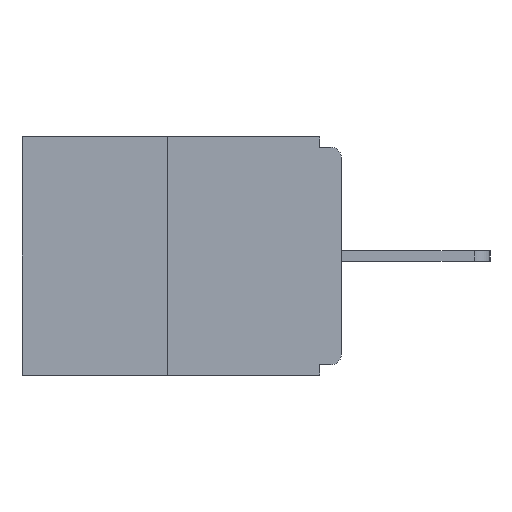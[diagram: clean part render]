
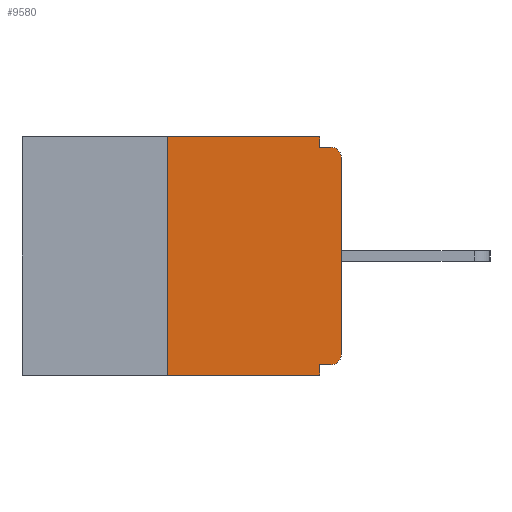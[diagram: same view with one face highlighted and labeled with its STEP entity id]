
A CAD part, left-side view. The second image highlights one B-rep face of the part: STEP entity #9580.
In plain terms, the highlighted planar face has unit normal (-1, 0, 0).
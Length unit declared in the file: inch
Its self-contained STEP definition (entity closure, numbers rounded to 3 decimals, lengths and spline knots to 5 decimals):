
#209 = DIRECTION ( 'NONE',  ( 0., 0., -1. ) ) ;
#618 = CIRCLE ( 'NONE', #10416, 0.015 ) ;
#1016 = CARTESIAN_POINT ( 'NONE',  ( 0., 0.25, 0. ) ) ;
#1125 = VERTEX_POINT ( 'NONE', #4318 ) ;
#2006 = VERTEX_POINT ( 'NONE', #5354 ) ;
#2096 = VECTOR ( 'NONE', #12347, 39.37008 ) ;
#3022 = CARTESIAN_POINT ( 'NONE',  ( 0., 0.015, -0.03 ) ) ;
#3151 = EDGE_CURVE ( 'NONE', #7987, #12108, #8639, .T. ) ;
#3240 = VECTOR ( 'NONE', #10092, 39.37008 ) ;
#3279 = CARTESIAN_POINT ( 'NONE',  ( 0., 0.46, 0. ) ) ;
#3523 = VECTOR ( 'NONE', #9205, 39.37008 ) ;
#3609 = VERTEX_POINT ( 'NONE', #15906 ) ;
#3686 = CIRCLE ( 'NONE', #14062, 0.015 ) ;
#3848 = DIRECTION ( 'NONE',  ( 0., 0., 1. ) ) ;
#3893 = EDGE_CURVE ( 'NONE', #3609, #7786, #13995, .T. ) ;
#4023 = ORIENTED_EDGE ( 'NONE', *, *, #7050, .F. ) ;
#4318 = CARTESIAN_POINT ( 'NONE',  ( 0., 0., -0.03 ) ) ;
#4526 = DIRECTION ( 'NONE',  ( 0., -1., 0. ) ) ;
#5007 = EDGE_CURVE ( 'NONE', #3609, #14325, #11975, .T. ) ;
#5299 = DIRECTION ( 'NONE',  ( 0., 0., -1. ) ) ;
#5317 = ORIENTED_EDGE ( 'NONE', *, *, #13819, .T. ) ;
#5354 = CARTESIAN_POINT ( 'NONE',  ( 0., 0., -0.313 ) ) ;
#5488 = CARTESIAN_POINT ( 'NONE',  ( 0., 0.031, -0.015 ) ) ;
#5637 = ORIENTED_EDGE ( 'NONE', *, *, #11343, .T. ) ;
#5960 = CARTESIAN_POINT ( 'NONE',  ( 0., 0.015, -0.313 ) ) ;
#6336 = ORIENTED_EDGE ( 'NONE', *, *, #13317, .F. ) ;
#6872 = ORIENTED_EDGE ( 'NONE', *, *, #14197, .F. ) ;
#6934 = VERTEX_POINT ( 'NONE', #7662 ) ;
#7050 = EDGE_CURVE ( 'NONE', #7243, #7786, #9281, .T. ) ;
#7098 = ORIENTED_EDGE ( 'NONE', *, *, #5007, .F. ) ;
#7243 = VERTEX_POINT ( 'NONE', #16182 ) ;
#7280 = DIRECTION ( 'NONE',  ( 0., 0., -1. ) ) ;
#7662 = CARTESIAN_POINT ( 'NONE',  ( 0., 0.015, -0.328 ) ) ;
#7786 = VERTEX_POINT ( 'NONE', #15159 ) ;
#7987 = VERTEX_POINT ( 'NONE', #16040 ) ;
#8366 = AXIS2_PLACEMENT_3D ( 'NONE', #17029, #15665, #7280 ) ;
#8455 = FACE_OUTER_BOUND ( 'NONE', #14030, .T. ) ;
#8561 = ORIENTED_EDGE ( 'NONE', *, *, #3893, .T. ) ;
#8586 = DIRECTION ( 'NONE',  ( -1., 0., 0. ) ) ;
#8639 = LINE ( 'NONE', #11357, #16052 ) ;
#9205 = DIRECTION ( 'NONE',  ( 0., 1., 0. ) ) ;
#9281 = LINE ( 'NONE', #12270, #11796 ) ;
#9580 = ADVANCED_FACE ( 'NONE', ( #8455 ), #11345, .F. ) ;
#9910 = LINE ( 'NONE', #16772, #3240 ) ;
#10092 = DIRECTION ( 'NONE',  ( 0., -1., 0. ) ) ;
#10416 = AXIS2_PLACEMENT_3D ( 'NONE', #5960, #8586, #13929 ) ;
#10555 = LINE ( 'NONE', #13081, #3523 ) ;
#10669 = VECTOR ( 'NONE', #3848, 39.37008 ) ;
#10733 = VECTOR ( 'NONE', #11379, 39.37008 ) ;
#10818 = CARTESIAN_POINT ( 'NONE',  ( 0., 0., 0. ) ) ;
#11236 = DIRECTION ( 'NONE',  ( -1., 0., 0. ) ) ;
#11289 = CARTESIAN_POINT ( 'NONE',  ( 0., 0.46, -0.343 ) ) ;
#11343 = EDGE_CURVE ( 'NONE', #6934, #2006, #618, .T. ) ;
#11345 = PLANE ( 'NONE',  #8366 ) ;
#11357 = CARTESIAN_POINT ( 'NONE',  ( 0., 0.031, 0. ) ) ;
#11379 = DIRECTION ( 'NONE',  ( 0., -1., 0. ) ) ;
#11381 = ORIENTED_EDGE ( 'NONE', *, *, #13637, .F. ) ;
#11796 = VECTOR ( 'NONE', #5299, 39.37008 ) ;
#11975 = LINE ( 'NONE', #16207, #10669 ) ;
#12108 = VERTEX_POINT ( 'NONE', #5488 ) ;
#12270 = CARTESIAN_POINT ( 'NONE',  ( 0., 0.031, -0.343 ) ) ;
#12347 = DIRECTION ( 'NONE',  ( 0., 0., 1. ) ) ;
#12496 = VECTOR ( 'NONE', #4526, 39.37008 ) ;
#13081 = CARTESIAN_POINT ( 'NONE',  ( 0., 0., -0.328 ) ) ;
#13226 = CARTESIAN_POINT ( 'NONE',  ( 0., 0.015, -0.015 ) ) ;
#13317 = EDGE_CURVE ( 'NONE', #6934, #7243, #10555, .T. ) ;
#13637 = EDGE_CURVE ( 'NONE', #12108, #15612, #9910, .T. ) ;
#13819 = EDGE_CURVE ( 'NONE', #2006, #1125, #17851, .T. ) ;
#13929 = DIRECTION ( 'NONE',  ( 0., 0., -1. ) ) ;
#13995 = LINE ( 'NONE', #11289, #10733 ) ;
#14030 = EDGE_LOOP ( 'NONE', ( #6872, #7098, #8561, #4023, #6336, #5637, #5317, #16307, #11381, #17110 ) ) ;
#14057 = DIRECTION ( 'NONE',  ( 0., 0., -1. ) ) ;
#14062 = AXIS2_PLACEMENT_3D ( 'NONE', #3022, #11236, #209 ) ;
#14197 = EDGE_CURVE ( 'NONE', #14325, #7987, #15909, .T. ) ;
#14325 = VERTEX_POINT ( 'NONE', #1016 ) ;
#15159 = CARTESIAN_POINT ( 'NONE',  ( 0., 0.031, -0.343 ) ) ;
#15612 = VERTEX_POINT ( 'NONE', #13226 ) ;
#15665 = DIRECTION ( 'NONE',  ( 1., 0., 0. ) ) ;
#15906 = CARTESIAN_POINT ( 'NONE',  ( 0., 0.25, -0.343 ) ) ;
#15909 = LINE ( 'NONE', #3279, #12496 ) ;
#16040 = CARTESIAN_POINT ( 'NONE',  ( 0., 0.031, 0. ) ) ;
#16052 = VECTOR ( 'NONE', #14057, 39.37008 ) ;
#16182 = CARTESIAN_POINT ( 'NONE',  ( 0., 0.031, -0.328 ) ) ;
#16207 = CARTESIAN_POINT ( 'NONE',  ( 0., 0.25, 0. ) ) ;
#16307 = ORIENTED_EDGE ( 'NONE', *, *, #17131, .T. ) ;
#16772 = CARTESIAN_POINT ( 'NONE',  ( 0., 0., -0.015 ) ) ;
#17029 = CARTESIAN_POINT ( 'NONE',  ( 0., 0.46, 0. ) ) ;
#17110 = ORIENTED_EDGE ( 'NONE', *, *, #3151, .F. ) ;
#17131 = EDGE_CURVE ( 'NONE', #1125, #15612, #3686, .T. ) ;
#17851 = LINE ( 'NONE', #10818, #2096 ) ;
